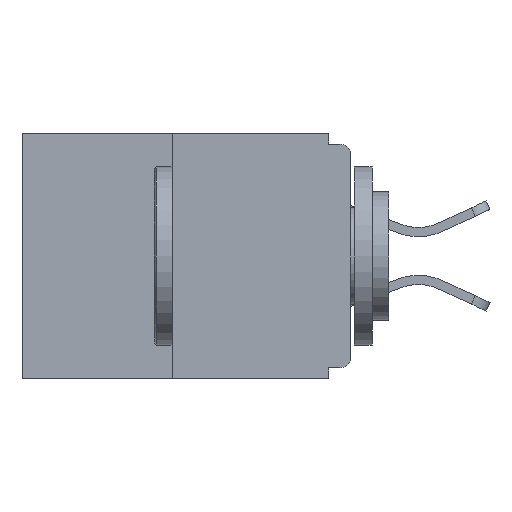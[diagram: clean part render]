
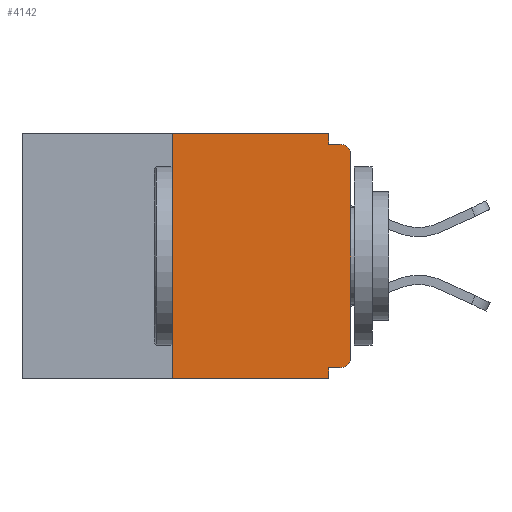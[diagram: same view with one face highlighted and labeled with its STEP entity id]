
A CAD part, left-side view. The second image highlights one B-rep face of the part: STEP entity #4142.
In plain terms, the highlighted planar face has unit normal (-1, 0, 0).
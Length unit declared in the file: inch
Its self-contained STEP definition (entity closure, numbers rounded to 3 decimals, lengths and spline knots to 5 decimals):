
#17 = LINE ( 'NONE', #5464, #20113 ) ;
#208 = CARTESIAN_POINT ( 'NONE',  ( 0., 0., -0.313 ) ) ;
#254 = CARTESIAN_POINT ( 'NONE',  ( 0., 0.25, 0. ) ) ;
#292 = ORIENTED_EDGE ( 'NONE', *, *, #768, .T. ) ;
#768 = EDGE_CURVE ( 'NONE', #4002, #12375, #12882, .T. ) ;
#1283 = VECTOR ( 'NONE', #14207, 39.37008 ) ;
#1346 = EDGE_CURVE ( 'NONE', #4002, #16226, #8601, .T. ) ;
#2270 = DIRECTION ( 'NONE',  ( 0., 0., -1. ) ) ;
#2913 = VERTEX_POINT ( 'NONE', #18754 ) ;
#2919 = CARTESIAN_POINT ( 'NONE',  ( 0., 0.46, -0.343 ) ) ;
#3329 = AXIS2_PLACEMENT_3D ( 'NONE', #19288, #8462, #13130 ) ;
#3367 = CARTESIAN_POINT ( 'NONE',  ( 0., 0.031, -0.343 ) ) ;
#3579 = LINE ( 'NONE', #20654, #1283 ) ;
#3664 = CARTESIAN_POINT ( 'NONE',  ( 0., 0., -0.03 ) ) ;
#3773 = ORIENTED_EDGE ( 'NONE', *, *, #4687, .T. ) ;
#4002 = VERTEX_POINT ( 'NONE', #19143 ) ;
#4142 = ADVANCED_FACE ( 'NONE', ( #15347 ), #6653, .F. ) ;
#4687 = EDGE_CURVE ( 'NONE', #12375, #9471, #3579, .T. ) ;
#4932 = DIRECTION ( 'NONE',  ( -1., 0., 0. ) ) ;
#5002 = VECTOR ( 'NONE', #16877, 39.37008 ) ;
#5310 = EDGE_CURVE ( 'NONE', #2913, #7844, #16833, .T. ) ;
#5464 = CARTESIAN_POINT ( 'NONE',  ( 0., 0.031, -0.343 ) ) ;
#5513 = VERTEX_POINT ( 'NONE', #10073 ) ;
#5519 = EDGE_CURVE ( 'NONE', #16226, #16820, #17, .T. ) ;
#6120 = EDGE_CURVE ( 'NONE', #7844, #5513, #10037, .T. ) ;
#6161 = DIRECTION ( 'NONE',  ( 0., -1., 0. ) ) ;
#6330 = CARTESIAN_POINT ( 'NONE',  ( 0., 0.015, -0.313 ) ) ;
#6382 = CARTESIAN_POINT ( 'NONE',  ( 0., 0.031, 0. ) ) ;
#6586 = DIRECTION ( 'NONE',  ( -1., 0., 0. ) ) ;
#6653 = PLANE ( 'NONE',  #3329 ) ;
#7015 = DIRECTION ( 'NONE',  ( 0., -1., 0. ) ) ;
#7421 = EDGE_CURVE ( 'NONE', #7670, #14125, #15718, .T. ) ;
#7569 = DIRECTION ( 'NONE',  ( 0., 1., 0. ) ) ;
#7670 = VERTEX_POINT ( 'NONE', #10082 ) ;
#7844 = VERTEX_POINT ( 'NONE', #16075 ) ;
#8284 = VECTOR ( 'NONE', #13626, 39.37008 ) ;
#8462 = DIRECTION ( 'NONE',  ( 1., 0., 0. ) ) ;
#8601 = LINE ( 'NONE', #17152, #11836 ) ;
#8905 = CARTESIAN_POINT ( 'NONE',  ( 0., 0., -0.015 ) ) ;
#8950 = EDGE_CURVE ( 'NONE', #9471, #5513, #10420, .T. ) ;
#9471 = VERTEX_POINT ( 'NONE', #3664 ) ;
#10037 = LINE ( 'NONE', #8905, #8284 ) ;
#10073 = CARTESIAN_POINT ( 'NONE',  ( 0., 0.015, -0.015 ) ) ;
#10082 = CARTESIAN_POINT ( 'NONE',  ( 0., 0.25, -0.343 ) ) ;
#10420 = CIRCLE ( 'NONE', #19138, 0.015 ) ;
#10435 = ORIENTED_EDGE ( 'NONE', *, *, #5519, .F. ) ;
#11034 = ORIENTED_EDGE ( 'NONE', *, *, #1346, .F. ) ;
#11836 = VECTOR ( 'NONE', #7569, 39.37008 ) ;
#11855 = DIRECTION ( 'NONE',  ( 0., 0., -1. ) ) ;
#12261 = AXIS2_PLACEMENT_3D ( 'NONE', #6330, #4932, #16093 ) ;
#12375 = VERTEX_POINT ( 'NONE', #208 ) ;
#12565 = LINE ( 'NONE', #16715, #19622 ) ;
#12761 = CARTESIAN_POINT ( 'NONE',  ( 0., 0.25, 0. ) ) ;
#12882 = CIRCLE ( 'NONE', #12261, 0.015 ) ;
#13006 = ORIENTED_EDGE ( 'NONE', *, *, #6120, .F. ) ;
#13130 = DIRECTION ( 'NONE',  ( 0., 0., -1. ) ) ;
#13352 = ORIENTED_EDGE ( 'NONE', *, *, #14307, .F. ) ;
#13406 = VECTOR ( 'NONE', #6161, 39.37008 ) ;
#13626 = DIRECTION ( 'NONE',  ( 0., -1., 0. ) ) ;
#14114 = ORIENTED_EDGE ( 'NONE', *, *, #8950, .T. ) ;
#14125 = VERTEX_POINT ( 'NONE', #254 ) ;
#14207 = DIRECTION ( 'NONE',  ( 0., 0., 1. ) ) ;
#14307 = EDGE_CURVE ( 'NONE', #14125, #2913, #12565, .T. ) ;
#14539 = CARTESIAN_POINT ( 'NONE',  ( 0., 0.015, -0.03 ) ) ;
#15347 = FACE_OUTER_BOUND ( 'NONE', #20149, .T. ) ;
#15684 = LINE ( 'NONE', #2919, #13406 ) ;
#15718 = LINE ( 'NONE', #12761, #5002 ) ;
#15952 = DIRECTION ( 'NONE',  ( 0., 0., -1. ) ) ;
#16075 = CARTESIAN_POINT ( 'NONE',  ( 0., 0.031, -0.015 ) ) ;
#16084 = VECTOR ( 'NONE', #15952, 39.37008 ) ;
#16093 = DIRECTION ( 'NONE',  ( 0., 0., -1. ) ) ;
#16149 = ORIENTED_EDGE ( 'NONE', *, *, #18762, .T. ) ;
#16226 = VERTEX_POINT ( 'NONE', #18599 ) ;
#16327 = ORIENTED_EDGE ( 'NONE', *, *, #5310, .F. ) ;
#16715 = CARTESIAN_POINT ( 'NONE',  ( 0., 0.46, 0. ) ) ;
#16820 = VERTEX_POINT ( 'NONE', #3367 ) ;
#16833 = LINE ( 'NONE', #6382, #16084 ) ;
#16877 = DIRECTION ( 'NONE',  ( 0., 0., 1. ) ) ;
#17152 = CARTESIAN_POINT ( 'NONE',  ( 0., 0., -0.328 ) ) ;
#17900 = ORIENTED_EDGE ( 'NONE', *, *, #7421, .F. ) ;
#18599 = CARTESIAN_POINT ( 'NONE',  ( 0., 0.031, -0.328 ) ) ;
#18754 = CARTESIAN_POINT ( 'NONE',  ( 0., 0.031, 0. ) ) ;
#18762 = EDGE_CURVE ( 'NONE', #7670, #16820, #15684, .T. ) ;
#19138 = AXIS2_PLACEMENT_3D ( 'NONE', #14539, #6586, #2270 ) ;
#19143 = CARTESIAN_POINT ( 'NONE',  ( 0., 0.015, -0.328 ) ) ;
#19288 = CARTESIAN_POINT ( 'NONE',  ( 0., 0.46, 0. ) ) ;
#19622 = VECTOR ( 'NONE', #7015, 39.37008 ) ;
#20113 = VECTOR ( 'NONE', #11855, 39.37008 ) ;
#20149 = EDGE_LOOP ( 'NONE', ( #13352, #17900, #16149, #10435, #11034, #292, #3773, #14114, #13006, #16327 ) ) ;
#20654 = CARTESIAN_POINT ( 'NONE',  ( 0., 0., 0. ) ) ;
